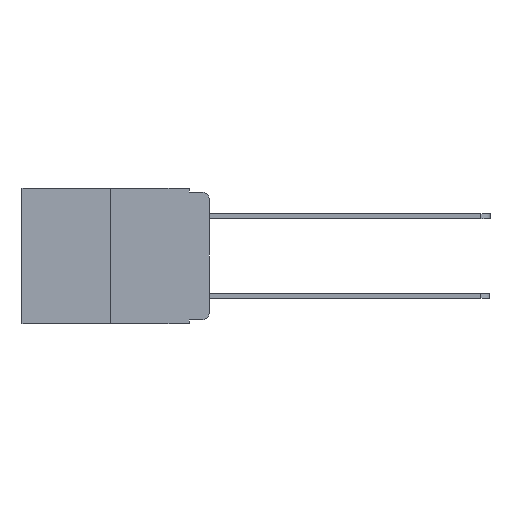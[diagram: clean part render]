
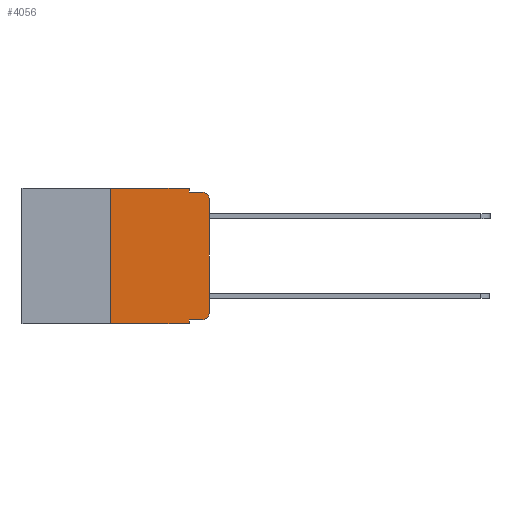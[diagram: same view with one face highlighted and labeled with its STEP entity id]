
A CAD part, left-side view. The second image highlights one B-rep face of the part: STEP entity #4056.
In plain terms, the highlighted planar face has unit normal (-1, 0, 0).
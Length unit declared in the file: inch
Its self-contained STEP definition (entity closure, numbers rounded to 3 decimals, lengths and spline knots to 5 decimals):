
#56 = ORIENTED_EDGE ( 'NONE', *, *, #7298, .T. ) ;
#60 = DIRECTION ( 'NONE',  ( 0., 0., 1. ) ) ;
#133 = ORIENTED_EDGE ( 'NONE', *, *, #1580, .T. ) ;
#154 = ORIENTED_EDGE ( 'NONE', *, *, #10252, .F. ) ;
#181 = CARTESIAN_POINT ( 'NONE',  ( 0., 0.051, 0. ) ) ;
#248 = VERTEX_POINT ( 'NONE', #726 ) ;
#314 = VECTOR ( 'NONE', #9912, 39.37008 ) ;
#457 = VERTEX_POINT ( 'NONE', #5887 ) ;
#726 = CARTESIAN_POINT ( 'NONE',  ( 0., 0.02, -0.01 ) ) ;
#746 = CARTESIAN_POINT ( 'NONE',  ( 0., 0.051, 0. ) ) ;
#876 = EDGE_CURVE ( 'NONE', #4237, #6501, #9148, .T. ) ;
#974 = CARTESIAN_POINT ( 'NONE',  ( 0., 0.25, -0.343 ) ) ;
#980 = ORIENTED_EDGE ( 'NONE', *, *, #876, .F. ) ;
#1048 = CARTESIAN_POINT ( 'NONE',  ( 0., 0., -0.313 ) ) ;
#1239 = DIRECTION ( 'NONE',  ( 0., -1., 0. ) ) ;
#1297 = ORIENTED_EDGE ( 'NONE', *, *, #5614, .F. ) ;
#1353 = CARTESIAN_POINT ( 'NONE',  ( 0., 0.051, -0.343 ) ) ;
#1440 = ORIENTED_EDGE ( 'NONE', *, *, #1497, .T. ) ;
#1497 = EDGE_CURVE ( 'NONE', #4237, #3328, #2897, .T. ) ;
#1547 = LINE ( 'NONE', #7764, #9583 ) ;
#1580 = EDGE_CURVE ( 'NONE', #1643, #6501, #6490, .T. ) ;
#1594 = DIRECTION ( 'NONE',  ( 0., 0., -1. ) ) ;
#1634 = VERTEX_POINT ( 'NONE', #1048 ) ;
#1643 = VERTEX_POINT ( 'NONE', #974 ) ;
#1651 = VERTEX_POINT ( 'NONE', #9487 ) ;
#1792 = ORIENTED_EDGE ( 'NONE', *, *, #2168, .T. ) ;
#2168 = EDGE_CURVE ( 'NONE', #3328, #1634, #9475, .T. ) ;
#2175 = CARTESIAN_POINT ( 'NONE',  ( 0., 0., -0.03 ) ) ;
#2850 = AXIS2_PLACEMENT_3D ( 'NONE', #7878, #3142, #8615 ) ;
#2897 = LINE ( 'NONE', #9378, #7181 ) ;
#3040 = CARTESIAN_POINT ( 'NONE',  ( 0., 0., 0. ) ) ;
#3064 = DIRECTION ( 'NONE',  ( 0., 0., -1. ) ) ;
#3142 = DIRECTION ( 'NONE',  ( -1., 0., 0. ) ) ;
#3210 = ORIENTED_EDGE ( 'NONE', *, *, #9764, .F. ) ;
#3328 = VERTEX_POINT ( 'NONE', #10082 ) ;
#3487 = LINE ( 'NONE', #6374, #7441 ) ;
#3523 = FACE_OUTER_BOUND ( 'NONE', #9740, .T. ) ;
#3910 = VERTEX_POINT ( 'NONE', #7396 ) ;
#4056 = ADVANCED_FACE ( 'NONE', ( #3523 ), #6261, .F. ) ;
#4237 = VERTEX_POINT ( 'NONE', #8267 ) ;
#4305 = LINE ( 'NONE', #181, #10038 ) ;
#4701 = DIRECTION ( 'NONE',  ( 0., 0., 1. ) ) ;
#4725 = CARTESIAN_POINT ( 'NONE',  ( 0., 0.473, 0. ) ) ;
#4924 = LINE ( 'NONE', #7444, #8428 ) ;
#5136 = DIRECTION ( 'NONE',  ( 0., 0., -1. ) ) ;
#5310 = DIRECTION ( 'NONE',  ( 1., 0., 0. ) ) ;
#5614 = EDGE_CURVE ( 'NONE', #3910, #1651, #4924, .T. ) ;
#5887 = CARTESIAN_POINT ( 'NONE',  ( 0., 0.051, -0.01 ) ) ;
#6229 = ORIENTED_EDGE ( 'NONE', *, *, #7781, .T. ) ;
#6261 = PLANE ( 'NONE',  #8759 ) ;
#6333 = DIRECTION ( 'NONE',  ( -1., 0., 0. ) ) ;
#6344 = CARTESIAN_POINT ( 'NONE',  ( 0., 0.02, -0.313 ) ) ;
#6374 = CARTESIAN_POINT ( 'NONE',  ( 0., 0.051, -0.01 ) ) ;
#6490 = LINE ( 'NONE', #10096, #314 ) ;
#6501 = VERTEX_POINT ( 'NONE', #1353 ) ;
#6686 = VECTOR ( 'NONE', #4701, 39.37008 ) ;
#6770 = DIRECTION ( 'NONE',  ( 0., 0., -1. ) ) ;
#6937 = ORIENTED_EDGE ( 'NONE', *, *, #8774, .F. ) ;
#7049 = DIRECTION ( 'NONE',  ( 0., -1., 0. ) ) ;
#7062 = VERTEX_POINT ( 'NONE', #2175 ) ;
#7135 = CIRCLE ( 'NONE', #2850, 0.02 ) ;
#7178 = VECTOR ( 'NONE', #1594, 39.37008 ) ;
#7181 = VECTOR ( 'NONE', #1239, 39.37008 ) ;
#7298 = EDGE_CURVE ( 'NONE', #1634, #7062, #8624, .T. ) ;
#7326 = DIRECTION ( 'NONE',  ( 0., -1., 0. ) ) ;
#7396 = CARTESIAN_POINT ( 'NONE',  ( 0., 0.25, 0. ) ) ;
#7441 = VECTOR ( 'NONE', #7049, 39.37008 ) ;
#7444 = CARTESIAN_POINT ( 'NONE',  ( 0., 0.473, 0. ) ) ;
#7764 = CARTESIAN_POINT ( 'NONE',  ( 0., 0.25, 0. ) ) ;
#7781 = EDGE_CURVE ( 'NONE', #7062, #248, #7135, .T. ) ;
#7878 = CARTESIAN_POINT ( 'NONE',  ( 0., 0.02, -0.03 ) ) ;
#8267 = CARTESIAN_POINT ( 'NONE',  ( 0., 0.051, -0.333 ) ) ;
#8428 = VECTOR ( 'NONE', #7326, 39.37008 ) ;
#8612 = AXIS2_PLACEMENT_3D ( 'NONE', #6344, #6333, #6770 ) ;
#8615 = DIRECTION ( 'NONE',  ( 0., 0., -1. ) ) ;
#8624 = LINE ( 'NONE', #3040, #6686 ) ;
#8759 = AXIS2_PLACEMENT_3D ( 'NONE', #4725, #5310, #5136 ) ;
#8774 = EDGE_CURVE ( 'NONE', #457, #248, #3487, .T. ) ;
#9148 = LINE ( 'NONE', #746, #7178 ) ;
#9378 = CARTESIAN_POINT ( 'NONE',  ( 0., 0.051, -0.333 ) ) ;
#9475 = CIRCLE ( 'NONE', #8612, 0.02 ) ;
#9487 = CARTESIAN_POINT ( 'NONE',  ( 0., 0.051, 0. ) ) ;
#9583 = VECTOR ( 'NONE', #60, 39.37008 ) ;
#9740 = EDGE_LOOP ( 'NONE', ( #56, #6229, #6937, #3210, #1297, #154, #133, #980, #1440, #1792 ) ) ;
#9764 = EDGE_CURVE ( 'NONE', #1651, #457, #4305, .T. ) ;
#9912 = DIRECTION ( 'NONE',  ( 0., -1., 0. ) ) ;
#10038 = VECTOR ( 'NONE', #3064, 39.37008 ) ;
#10082 = CARTESIAN_POINT ( 'NONE',  ( 0., 0.02, -0.333 ) ) ;
#10096 = CARTESIAN_POINT ( 'NONE',  ( 0., 0.473, -0.343 ) ) ;
#10252 = EDGE_CURVE ( 'NONE', #1643, #3910, #1547, .T. ) ;
